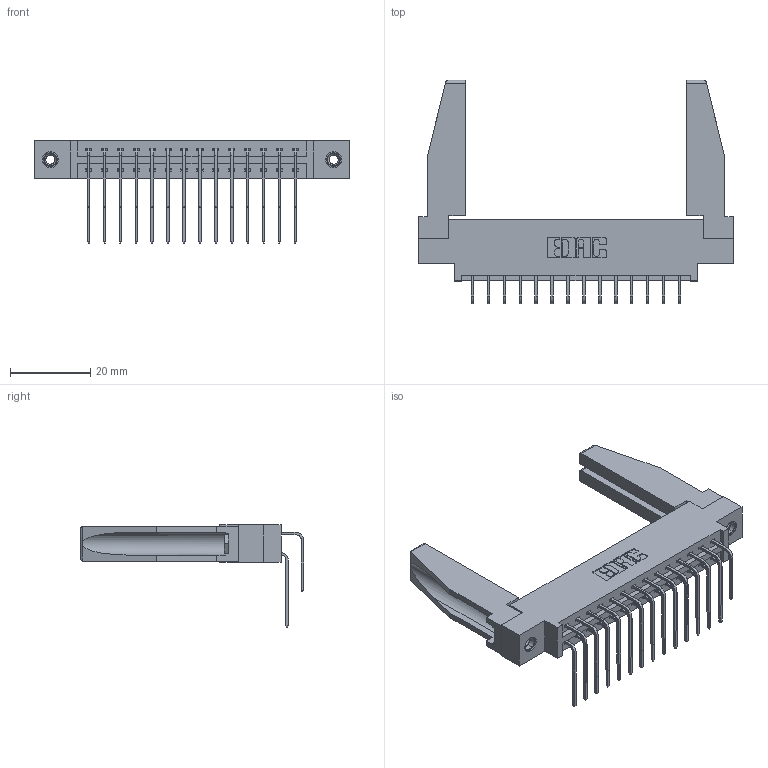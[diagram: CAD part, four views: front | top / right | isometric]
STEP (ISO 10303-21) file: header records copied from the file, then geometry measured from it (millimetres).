
FILE_DESCRIPTION (( 'STEP AP203' ), '1' );
FILE_NAME ('337-028-559-878.STEP', '2019-10-10T23:13:48', ( '' ), ( '' ), 'SwSTEP 2.0', 'SolidWorks 2016', '' );
FILE_SCHEMA (( 'CONFIG_CONTROL_DESIGN' ));
Length unit declared in the file: inch
Products named in the file (6): 307-220-078; 345-292-001_558 559 Tail - 1; 337 Part_0.170 Offset - 0.156 Dia-TI; 345-250-001_345-250-001-102; 337-028-559-878; 345-292-001_559 Tail - 2
Assembly tree (33 placements, depth 2):
  337-028-559-878
    337 Part_0.170 Offset - 0.156 Dia-TI
    345-292-001_558 559 Tail - 1  x14
    345-292-001_559 Tail - 2  x14
    345-250-001_345-250-001-102  x2
    307-220-078  x2
Bounding box: 78.49 x 55.69 x 25.53 mm (x, y, z)
Volume: 11936.1 mm3; surface area: 13456.7 mm2
Topology: 33 solids, 33 shells, 1816 faces, 5329 edges, 3506 vertices
Faces by surface type: plane 1278, cylinder 522, cone 12, torus 4
Entity records: 18832 total; most frequent: CARTESIAN_POINT 3243, ORIENTED_EDGE 3084, DIRECTION 2798, EDGE_CURVE 1542, LINE 1336, VECTOR 1336, VERTEX_POINT 1020, AXIS2_PLACEMENT_3D 731
